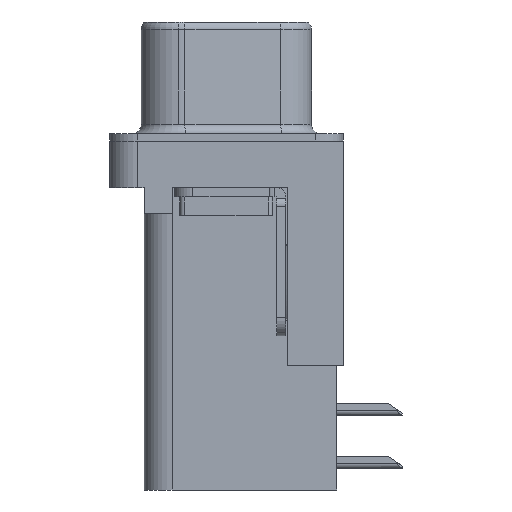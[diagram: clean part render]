
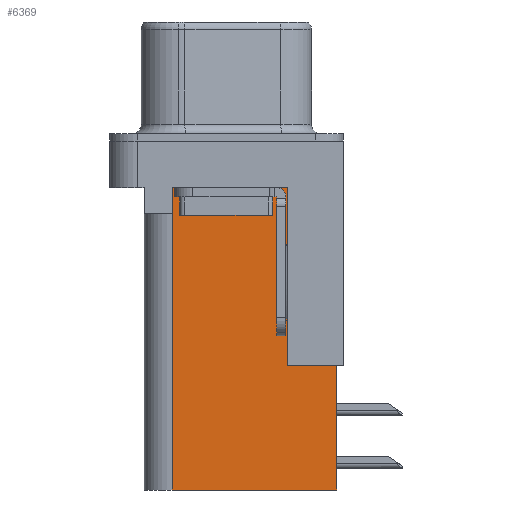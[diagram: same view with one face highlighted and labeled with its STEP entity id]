
A CAD part, left-side view. The second image highlights one B-rep face of the part: STEP entity #6369.
In plain terms, the highlighted planar face has unit normal (-1, 0, 0).
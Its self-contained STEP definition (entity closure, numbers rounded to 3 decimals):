
#194 = LINE ( 'NONE', #3249, #15068 ) ;
#228 = CARTESIAN_POINT ( 'NONE',  ( 3.765, -3.295, -12.05 ) ) ;
#334 = EDGE_CURVE ( 'NONE', #5995, #1252, #194, .T. ) ;
#798 = EDGE_CURVE ( 'NONE', #8599, #12959, #1530, .T. ) ;
#866 = LINE ( 'NONE', #13819, #11877 ) ;
#1014 = CARTESIAN_POINT ( 'NONE',  ( 3.765, 2.925, -3.9 ) ) ;
#1252 = VERTEX_POINT ( 'NONE', #1014 ) ;
#1317 = CARTESIAN_POINT ( 'NONE',  ( 3.765, -6.295, -12.05 ) ) ;
#1530 = LINE ( 'NONE', #9608, #16393 ) ;
#3249 = CARTESIAN_POINT ( 'NONE',  ( 3.765, 2.925, -18.76 ) ) ;
#3403 = ORIENTED_EDGE ( 'NONE', *, *, #7488, .F. ) ;
#4647 = FACE_OUTER_BOUND ( 'NONE', #10106, .T. ) ;
#4845 = CARTESIAN_POINT ( 'NONE',  ( 3.765, -5.925, -12.05 ) ) ;
#4962 = DIRECTION ( 'NONE',  ( 0., 1., 0. ) ) ;
#5325 = EDGE_CURVE ( 'NONE', #12959, #1252, #866, .T. ) ;
#5423 = LINE ( 'NONE', #16684, #16922 ) ;
#5498 = DIRECTION ( 'NONE',  ( 0., 1., 0. ) ) ;
#5573 = CARTESIAN_POINT ( 'NONE',  ( 3.765, 2.895, -3.9 ) ) ;
#5645 = LINE ( 'NONE', #1317, #9442 ) ;
#5889 = ORIENTED_EDGE ( 'NONE', *, *, #9329, .T. ) ;
#5995 = VERTEX_POINT ( 'NONE', #12750 ) ;
#5997 = ORIENTED_EDGE ( 'NONE', *, *, #334, .F. ) ;
#6258 = CARTESIAN_POINT ( 'NONE',  ( 3.765, -3.295, -18.76 ) ) ;
#6369 = ADVANCED_FACE ( 'NONE', ( #4647 ), #14859, .F. ) ;
#6597 = CARTESIAN_POINT ( 'NONE',  ( 3.765, 2.895, -2.5 ) ) ;
#7073 = LINE ( 'NONE', #9633, #18093 ) ;
#7479 = VECTOR ( 'NONE', #5498, 1000. ) ;
#7488 = EDGE_CURVE ( 'NONE', #9694, #10887, #7073, .T. ) ;
#7724 = DIRECTION ( 'NONE',  ( 0., 1., 0. ) ) ;
#8373 = AXIS2_PLACEMENT_3D ( 'NONE', #6258, #16363, #7724 ) ;
#8599 = VERTEX_POINT ( 'NONE', #6597 ) ;
#8895 = VERTEX_POINT ( 'NONE', #228 ) ;
#8941 = ORIENTED_EDGE ( 'NONE', *, *, #17987, .T. ) ;
#9329 = EDGE_CURVE ( 'NONE', #12965, #8599, #11325, .T. ) ;
#9441 = CARTESIAN_POINT ( 'NONE',  ( 3.765, -5.925, -18.76 ) ) ;
#9442 = VECTOR ( 'NONE', #11366, 1000. ) ;
#9608 = CARTESIAN_POINT ( 'NONE',  ( 3.765, 2.895, -3.9 ) ) ;
#9633 = CARTESIAN_POINT ( 'NONE',  ( 3.765, -5.925, -2. ) ) ;
#9694 = VERTEX_POINT ( 'NONE', #4845 ) ;
#10067 = VECTOR ( 'NONE', #4962, 1000. ) ;
#10106 = EDGE_LOOP ( 'NONE', ( #5889, #12205, #14163, #5997, #14303, #3403, #8941, #14644 ) ) ;
#10755 = EDGE_CURVE ( 'NONE', #8895, #12965, #5423, .T. ) ;
#10887 = VERTEX_POINT ( 'NONE', #9441 ) ;
#11325 = LINE ( 'NONE', #15586, #7479 ) ;
#11366 = DIRECTION ( 'NONE',  ( 0., 1., 0. ) ) ;
#11877 = VECTOR ( 'NONE', #16713, 1000. ) ;
#12197 = EDGE_CURVE ( 'NONE', #10887, #5995, #13942, .T. ) ;
#12205 = ORIENTED_EDGE ( 'NONE', *, *, #798, .T. ) ;
#12750 = CARTESIAN_POINT ( 'NONE',  ( 3.765, 2.925, -18.76 ) ) ;
#12829 = CARTESIAN_POINT ( 'NONE',  ( 3.765, -3.295, -2.5 ) ) ;
#12959 = VERTEX_POINT ( 'NONE', #5573 ) ;
#12965 = VERTEX_POINT ( 'NONE', #12829 ) ;
#13819 = CARTESIAN_POINT ( 'NONE',  ( 3.765, 0., -3.9 ) ) ;
#13942 = LINE ( 'NONE', #16427, #10067 ) ;
#14163 = ORIENTED_EDGE ( 'NONE', *, *, #5325, .T. ) ;
#14303 = ORIENTED_EDGE ( 'NONE', *, *, #12197, .F. ) ;
#14639 = DIRECTION ( 'NONE',  ( 0., 0., -1. ) ) ;
#14644 = ORIENTED_EDGE ( 'NONE', *, *, #10755, .T. ) ;
#14859 = PLANE ( 'NONE',  #8373 ) ;
#15068 = VECTOR ( 'NONE', #15249, 1000. ) ;
#15249 = DIRECTION ( 'NONE',  ( 0., 0., 1. ) ) ;
#15586 = CARTESIAN_POINT ( 'NONE',  ( 3.765, -3.295, -2.5 ) ) ;
#16363 = DIRECTION ( 'NONE',  ( 1., 0., 0. ) ) ;
#16393 = VECTOR ( 'NONE', #14639, 1000. ) ;
#16427 = CARTESIAN_POINT ( 'NONE',  ( 3.765, -3.295, -18.76 ) ) ;
#16684 = CARTESIAN_POINT ( 'NONE',  ( 3.765, -3.295, -18.76 ) ) ;
#16713 = DIRECTION ( 'NONE',  ( 0., 1., 0. ) ) ;
#16847 = DIRECTION ( 'NONE',  ( 0., 0., -1. ) ) ;
#16922 = VECTOR ( 'NONE', #18047, 1000. ) ;
#17987 = EDGE_CURVE ( 'NONE', #9694, #8895, #5645, .T. ) ;
#18047 = DIRECTION ( 'NONE',  ( 0., 0., 1. ) ) ;
#18093 = VECTOR ( 'NONE', #16847, 1000. ) ;
